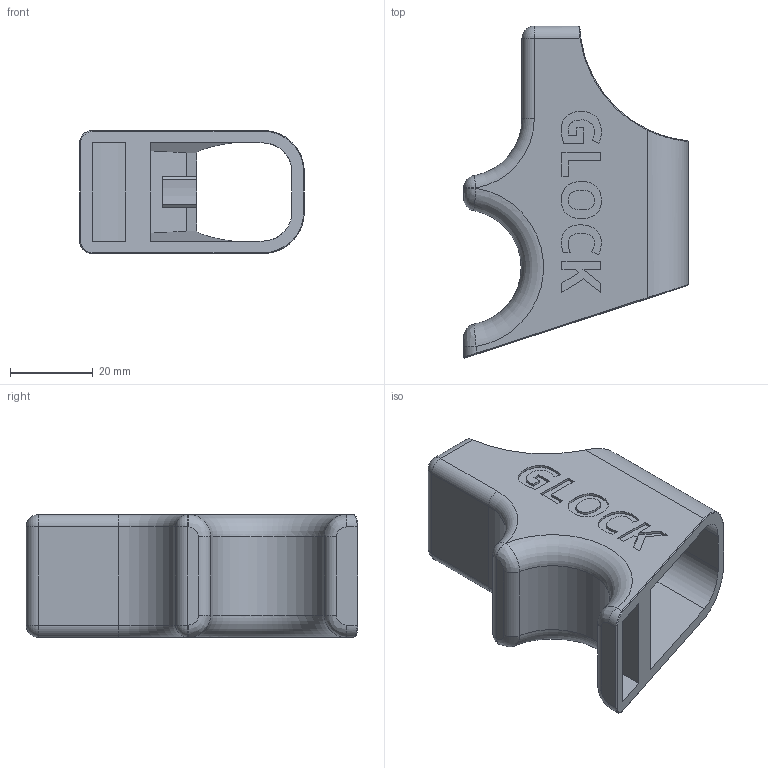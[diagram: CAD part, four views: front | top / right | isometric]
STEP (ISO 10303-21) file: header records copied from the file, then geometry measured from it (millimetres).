
FILE_DESCRIPTION(/* description */ (''),/* implementation_level */ '2;1');
FILE_NAME(/* name */ '5fc6b1f7b754c810bf2c6067',/* time_stamp */ '2020-12-01T21:13:28+00:00',/* author */ (''),/* organization */ (''),/* preprocessor_version */ 'ST-DEVELOPER v16.7',/* originating_system */ $,/* authorisation */ $);
FILE_SCHEMA (('AUTOMOTIVE_DESIGN {1 0 10303 214 3 1 1}'));
Length unit declared in the file: metre
Products named in the file (1): Glock Magazine Loader V1.6.3
Bounding box: 54.41 x 80.38 x 29.75 mm (x, y, z)
Volume: 30544.1 mm3; surface area: 17072.2 mm2
Topology: 1 solids, 1 shells, 151 faces, 388 edges, 244 vertices
Faces by surface type: plane 68, bspline 53, cylinder 20, torus 4, sphere 4, cone 2
Entity records: 4997 total; most frequent: CARTESIAN_POINT 1694, ORIENTED_EDGE 772, DIRECTION 502, EDGE_CURVE 386, VERTEX_POINT 244, LINE 220, VECTOR 220, EDGE_LOOP 160
